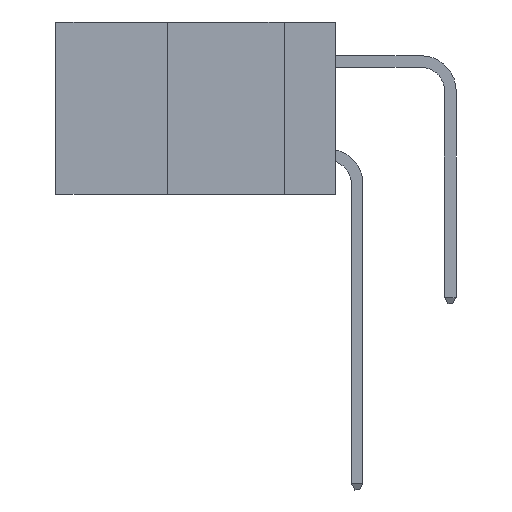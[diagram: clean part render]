
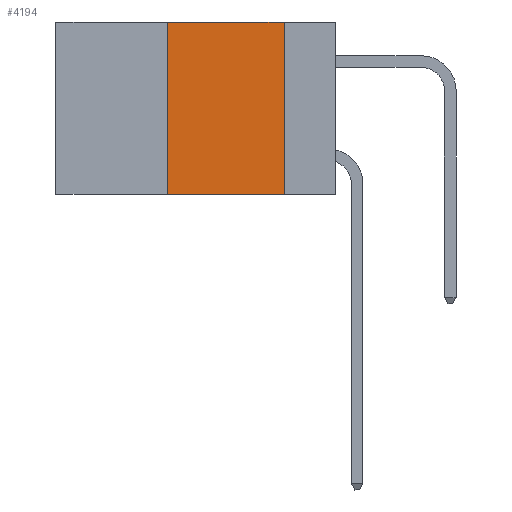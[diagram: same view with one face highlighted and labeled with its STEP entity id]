
A CAD part, left-side view. The second image highlights one B-rep face of the part: STEP entity #4194.
In plain terms, the highlighted planar face has unit normal (-1, 0, 0).
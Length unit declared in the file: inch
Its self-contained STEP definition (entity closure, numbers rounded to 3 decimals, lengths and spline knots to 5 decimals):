
#57 = VERTEX_POINT ( 'NONE', #2060 ) ;
#167 = VERTEX_POINT ( 'NONE', #759 ) ;
#626 = LINE ( 'NONE', #4093, #3782 ) ;
#759 = CARTESIAN_POINT ( 'NONE',  ( 0., 0.11, -0.37 ) ) ;
#1501 = EDGE_CURVE ( 'NONE', #57, #167, #2242, .T. ) ;
#2060 = CARTESIAN_POINT ( 'NONE',  ( 0., 0.11, 0. ) ) ;
#2242 = LINE ( 'NONE', #6659, #12814 ) ;
#2383 = LINE ( 'NONE', #7888, #9361 ) ;
#2929 = PLANE ( 'NONE',  #11555 ) ;
#3782 = VECTOR ( 'NONE', #5446, 39.37008 ) ;
#3818 = ORIENTED_EDGE ( 'NONE', *, *, #5032, .T. ) ;
#4093 = CARTESIAN_POINT ( 'NONE',  ( 0., 0.36, 0. ) ) ;
#4194 = ADVANCED_FACE ( 'NONE', ( #5704 ), #2929, .F. ) ;
#4366 = DIRECTION ( 'NONE',  ( 0., 0., -1. ) ) ;
#4491 = DIRECTION ( 'NONE',  ( 0., 0., -1. ) ) ;
#5032 = EDGE_CURVE ( 'NONE', #15776, #167, #6513, .T. ) ;
#5446 = DIRECTION ( 'NONE',  ( 0., 0., 1. ) ) ;
#5704 = FACE_OUTER_BOUND ( 'NONE', #7190, .T. ) ;
#6217 = ORIENTED_EDGE ( 'NONE', *, *, #1501, .F. ) ;
#6513 = LINE ( 'NONE', #9032, #16821 ) ;
#6659 = CARTESIAN_POINT ( 'NONE',  ( 0., 0.11, 0. ) ) ;
#7190 = EDGE_LOOP ( 'NONE', ( #6217, #9867, #17375, #3818 ) ) ;
#7888 = CARTESIAN_POINT ( 'NONE',  ( 0., 0.6, 0. ) ) ;
#8397 = EDGE_CURVE ( 'NONE', #15776, #17646, #626, .T. ) ;
#8483 = CARTESIAN_POINT ( 'NONE',  ( 0., 0.6, 0. ) ) ;
#9032 = CARTESIAN_POINT ( 'NONE',  ( 0., 0.6, -0.37 ) ) ;
#9361 = VECTOR ( 'NONE', #11906, 39.37008 ) ;
#9827 = EDGE_CURVE ( 'NONE', #17646, #57, #2383, .T. ) ;
#9867 = ORIENTED_EDGE ( 'NONE', *, *, #9827, .F. ) ;
#11555 = AXIS2_PLACEMENT_3D ( 'NONE', #8483, #12564, #4366 ) ;
#11906 = DIRECTION ( 'NONE',  ( 0., -1., 0. ) ) ;
#12564 = DIRECTION ( 'NONE',  ( 1., 0., 0. ) ) ;
#12814 = VECTOR ( 'NONE', #4491, 39.37008 ) ;
#13111 = DIRECTION ( 'NONE',  ( 0., -1., 0. ) ) ;
#13666 = CARTESIAN_POINT ( 'NONE',  ( 0., 0.36, -0.37 ) ) ;
#15570 = CARTESIAN_POINT ( 'NONE',  ( 0., 0.36, 0. ) ) ;
#15776 = VERTEX_POINT ( 'NONE', #13666 ) ;
#16821 = VECTOR ( 'NONE', #13111, 39.37008 ) ;
#17375 = ORIENTED_EDGE ( 'NONE', *, *, #8397, .F. ) ;
#17646 = VERTEX_POINT ( 'NONE', #15570 ) ;
